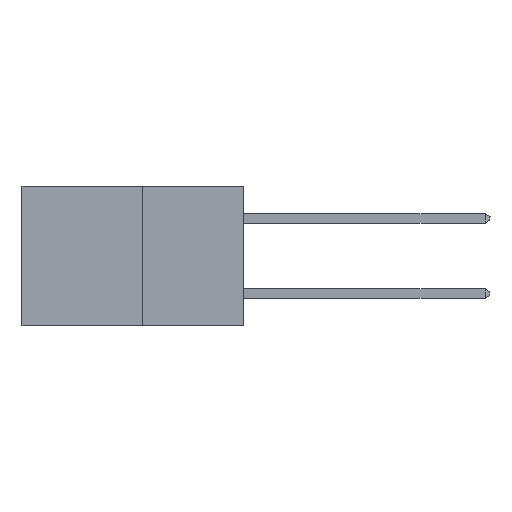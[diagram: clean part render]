
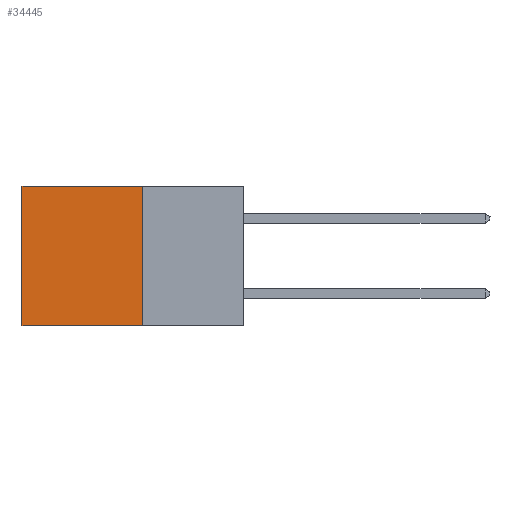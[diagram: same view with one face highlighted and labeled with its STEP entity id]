
A CAD part, left-side view. The second image highlights one B-rep face of the part: STEP entity #34445.
In plain terms, the highlighted planar face has unit normal (-1, 0, 0).
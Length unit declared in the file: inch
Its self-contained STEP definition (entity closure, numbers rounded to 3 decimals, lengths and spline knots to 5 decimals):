
#365 = VERTEX_POINT ( 'NONE', #8929 ) ;
#848 = VERTEX_POINT ( 'NONE', #13134 ) ;
#1071 = VECTOR ( 'NONE', #31610, 39.37008 ) ;
#1130 = CARTESIAN_POINT ( 'NONE',  ( 0.277, 0.27, -0.37 ) ) ;
#2523 = FACE_OUTER_BOUND ( 'NONE', #13699, .T. ) ;
#2827 = LINE ( 'NONE', #15378, #1071 ) ;
#4188 = VECTOR ( 'NONE', #14330, 39.37008 ) ;
#5067 = LINE ( 'NONE', #6312, #4188 ) ;
#6312 = CARTESIAN_POINT ( 'NONE',  ( 0.277, 0.27, 0. ) ) ;
#7101 = CARTESIAN_POINT ( 'NONE',  ( 0.277, 0.59, -0.37 ) ) ;
#7299 = EDGE_CURVE ( 'NONE', #365, #848, #5067, .T. ) ;
#7810 = LINE ( 'NONE', #1130, #13287 ) ;
#8036 = EDGE_CURVE ( 'NONE', #848, #10158, #2827, .T. ) ;
#8929 = CARTESIAN_POINT ( 'NONE',  ( 0.277, 0.27, 0. ) ) ;
#10158 = VERTEX_POINT ( 'NONE', #7101 ) ;
#10179 = EDGE_CURVE ( 'NONE', #14348, #10158, #31272, .T. ) ;
#11842 = PLANE ( 'NONE',  #23545 ) ;
#12011 = EDGE_CURVE ( 'NONE', #365, #14348, #7810, .T. ) ;
#13134 = CARTESIAN_POINT ( 'NONE',  ( 0.277, 0.59, 0. ) ) ;
#13287 = VECTOR ( 'NONE', #25808, 39.37008 ) ;
#13699 = EDGE_LOOP ( 'NONE', ( #22908, #22972, #23201, #21766 ) ) ;
#14330 = DIRECTION ( 'NONE',  ( 0., 1., 0. ) ) ;
#14348 = VERTEX_POINT ( 'NONE', #24043 ) ;
#14594 = DIRECTION ( 'NONE',  ( 1., 0., 0. ) ) ;
#15378 = CARTESIAN_POINT ( 'NONE',  ( 0.277, 0.59, -0.37 ) ) ;
#20876 = CARTESIAN_POINT ( 'NONE',  ( 0.277, 0.27, -0.37 ) ) ;
#21766 = ORIENTED_EDGE ( 'NONE', *, *, #7299, .T. ) ;
#22908 = ORIENTED_EDGE ( 'NONE', *, *, #8036, .T. ) ;
#22972 = ORIENTED_EDGE ( 'NONE', *, *, #10179, .F. ) ;
#23201 = ORIENTED_EDGE ( 'NONE', *, *, #12011, .F. ) ;
#23545 = AXIS2_PLACEMENT_3D ( 'NONE', #30875, #14594, #33503 ) ;
#24043 = CARTESIAN_POINT ( 'NONE',  ( 0.277, 0.27, -0.37 ) ) ;
#25808 = DIRECTION ( 'NONE',  ( 0., 0., -1. ) ) ;
#28795 = VECTOR ( 'NONE', #29076, 39.37008 ) ;
#29076 = DIRECTION ( 'NONE',  ( 0., 1., 0. ) ) ;
#30875 = CARTESIAN_POINT ( 'NONE',  ( 0.277, 0.27, -0.37 ) ) ;
#31272 = LINE ( 'NONE', #20876, #28795 ) ;
#31610 = DIRECTION ( 'NONE',  ( 0., 0., -1. ) ) ;
#33503 = DIRECTION ( 'NONE',  ( 0., 0., -1. ) ) ;
#34445 = ADVANCED_FACE ( 'NONE', ( #2523 ), #11842, .F. ) ;
